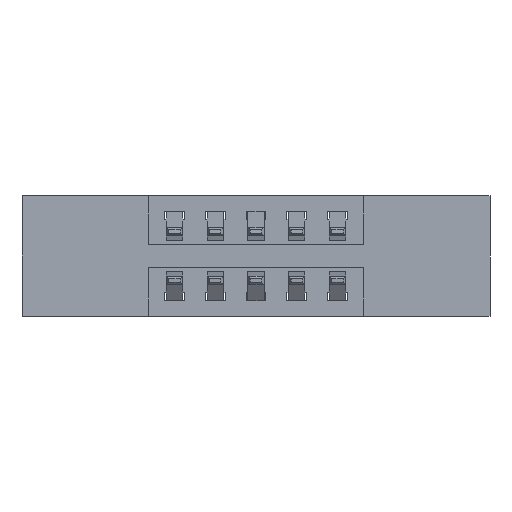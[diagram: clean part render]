
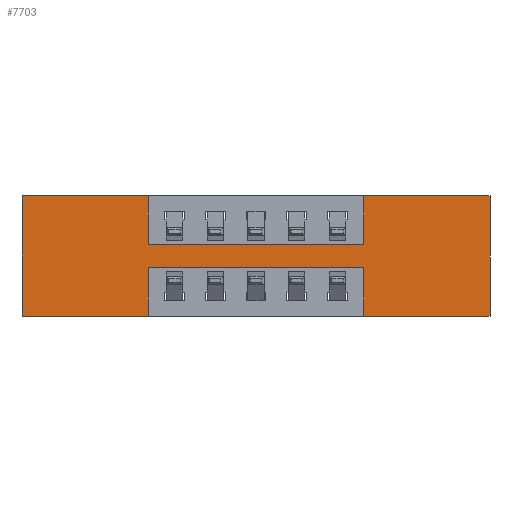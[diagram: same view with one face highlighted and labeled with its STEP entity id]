
A CAD part, front view. The second image highlights one B-rep face of the part: STEP entity #7703.
In plain terms, the highlighted planar face has unit normal (0, -1, 0).
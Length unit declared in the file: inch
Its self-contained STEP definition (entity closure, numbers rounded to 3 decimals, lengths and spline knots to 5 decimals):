
#15 = LINE ( 'NONE', #3158, #5585 ) ;
#16 = LINE ( 'NONE', #4874, #6699 ) ;
#152 = DIRECTION ( 'NONE',  ( 0., 0., 1. ) ) ;
#256 = EDGE_CURVE ( 'NONE', #5467, #5244, #16, .T. ) ;
#348 = ORIENTED_EDGE ( 'NONE', *, *, #256, .F. ) ;
#552 = CARTESIAN_POINT ( 'NONE',  ( 0.3875, 0., -0.22 ) ) ;
#829 = CARTESIAN_POINT ( 'NONE',  ( 0.3875, 0., 0. ) ) ;
#909 = LINE ( 'NONE', #829, #4134 ) ;
#952 = VERTEX_POINT ( 'NONE', #2493 ) ;
#1037 = DIRECTION ( 'NONE',  ( 1., 0., 0. ) ) ;
#1097 = ORIENTED_EDGE ( 'NONE', *, *, #2027, .F. ) ;
#1141 = CARTESIAN_POINT ( 'NONE',  ( 0., 0., 0. ) ) ;
#1165 = DIRECTION ( 'NONE',  ( -1., 0., 0. ) ) ;
#1270 = DIRECTION ( 'NONE',  ( 0., 0., -1. ) ) ;
#1451 = EDGE_CURVE ( 'NONE', #5244, #6331, #2304, .T. ) ;
#1646 = CARTESIAN_POINT ( 'NONE',  ( 0.3875, 0., -0.15 ) ) ;
#1742 = CARTESIAN_POINT ( 'NONE',  ( 0.3875, 0., -0.15 ) ) ;
#1752 = ORIENTED_EDGE ( 'NONE', *, *, #5271, .F. ) ;
#1842 = CARTESIAN_POINT ( 'NONE',  ( 1.435, 0., 0. ) ) ;
#1938 = CARTESIAN_POINT ( 'NONE',  ( 0., 0., -0.37 ) ) ;
#1953 = ORIENTED_EDGE ( 'NONE', *, *, #7779, .F. ) ;
#1957 = EDGE_LOOP ( 'NONE', ( #1752, #4332, #4628, #5695, #2259, #348, #4533, #7450, #1097, #2049, #7963, #1953 ) ) ;
#2027 = EDGE_CURVE ( 'NONE', #952, #4006, #909, .T. ) ;
#2049 = ORIENTED_EDGE ( 'NONE', *, *, #7031, .F. ) ;
#2076 = EDGE_CURVE ( 'NONE', #6331, #2893, #7748, .T. ) ;
#2101 = LINE ( 'NONE', #552, #5408 ) ;
#2259 = ORIENTED_EDGE ( 'NONE', *, *, #1451, .F. ) ;
#2304 = LINE ( 'NONE', #5465, #8083 ) ;
#2493 = CARTESIAN_POINT ( 'NONE',  ( 0.3875, 0., 0. ) ) ;
#2503 = DIRECTION ( 'NONE',  ( 0., -1., 0. ) ) ;
#2518 = LINE ( 'NONE', #1646, #4166 ) ;
#2599 = CARTESIAN_POINT ( 'NONE',  ( 0., 0., 0. ) ) ;
#2680 = CARTESIAN_POINT ( 'NONE',  ( 0., 0., -0.37 ) ) ;
#2754 = EDGE_CURVE ( 'NONE', #7626, #5467, #3765, .T. ) ;
#2893 = VERTEX_POINT ( 'NONE', #3043 ) ;
#2971 = VECTOR ( 'NONE', #152, 39.37008 ) ;
#3023 = CARTESIAN_POINT ( 'NONE',  ( 0.3875, 0., -0.22 ) ) ;
#3043 = CARTESIAN_POINT ( 'NONE',  ( 1.0475, 0., -0.37 ) ) ;
#3052 = DIRECTION ( 'NONE',  ( 0., 0., -1. ) ) ;
#3154 = CARTESIAN_POINT ( 'NONE',  ( 1.0475, 0., 0. ) ) ;
#3158 = CARTESIAN_POINT ( 'NONE',  ( 0., 0., -0.37 ) ) ;
#3169 = DIRECTION ( 'NONE',  ( 1., 0., 0. ) ) ;
#3387 = EDGE_CURVE ( 'NONE', #4006, #7626, #2518, .T. ) ;
#3481 = DIRECTION ( 'NONE',  ( 0., 0., -1. ) ) ;
#3765 = LINE ( 'NONE', #3154, #2971 ) ;
#3813 = EDGE_CURVE ( 'NONE', #2893, #7390, #5056, .T. ) ;
#3901 = VERTEX_POINT ( 'NONE', #6393 ) ;
#4006 = VERTEX_POINT ( 'NONE', #1742 ) ;
#4080 = DIRECTION ( 'NONE',  ( 0., 0., 1. ) ) ;
#4114 = VECTOR ( 'NONE', #7170, 39.37008 ) ;
#4128 = VECTOR ( 'NONE', #3481, 39.37008 ) ;
#4134 = VECTOR ( 'NONE', #3052, 39.37008 ) ;
#4166 = VECTOR ( 'NONE', #6750, 39.37008 ) ;
#4255 = VECTOR ( 'NONE', #4080, 39.37008 ) ;
#4318 = VECTOR ( 'NONE', #3169, 39.37008 ) ;
#4332 = ORIENTED_EDGE ( 'NONE', *, *, #5857, .F. ) ;
#4336 = LINE ( 'NONE', #8113, #4128 ) ;
#4382 = FACE_OUTER_BOUND ( 'NONE', #1957, .T. ) ;
#4533 = ORIENTED_EDGE ( 'NONE', *, *, #2754, .F. ) ;
#4628 = ORIENTED_EDGE ( 'NONE', *, *, #3813, .F. ) ;
#4759 = CARTESIAN_POINT ( 'NONE',  ( 1.435, 0., -0.37 ) ) ;
#4863 = CARTESIAN_POINT ( 'NONE',  ( 0., 0., 0. ) ) ;
#4874 = CARTESIAN_POINT ( 'NONE',  ( 0., 0., 0. ) ) ;
#4941 = VERTEX_POINT ( 'NONE', #3023 ) ;
#5006 = VERTEX_POINT ( 'NONE', #1141 ) ;
#5056 = LINE ( 'NONE', #6075, #4255 ) ;
#5075 = CARTESIAN_POINT ( 'NONE',  ( 0., 0., -0.37 ) ) ;
#5244 = VERTEX_POINT ( 'NONE', #1842 ) ;
#5271 = EDGE_CURVE ( 'NONE', #4941, #3901, #4336, .T. ) ;
#5408 = VECTOR ( 'NONE', #5653, 39.37008 ) ;
#5436 = DIRECTION ( 'NONE',  ( 0., 0., 1. ) ) ;
#5465 = CARTESIAN_POINT ( 'NONE',  ( 1.435, 0., 0. ) ) ;
#5467 = VERTEX_POINT ( 'NONE', #6349 ) ;
#5585 = VECTOR ( 'NONE', #1165, 39.37008 ) ;
#5653 = DIRECTION ( 'NONE',  ( -1., 0., 0. ) ) ;
#5667 = PLANE ( 'NONE',  #7977 ) ;
#5695 = ORIENTED_EDGE ( 'NONE', *, *, #2076, .F. ) ;
#5857 = EDGE_CURVE ( 'NONE', #7390, #4941, #2101, .T. ) ;
#5869 = VERTEX_POINT ( 'NONE', #5075 ) ;
#6075 = CARTESIAN_POINT ( 'NONE',  ( 1.0475, 0., -0.37 ) ) ;
#6229 = LINE ( 'NONE', #2599, #4318 ) ;
#6331 = VERTEX_POINT ( 'NONE', #4759 ) ;
#6349 = CARTESIAN_POINT ( 'NONE',  ( 1.0475, 0., 0. ) ) ;
#6393 = CARTESIAN_POINT ( 'NONE',  ( 0.3875, 0., -0.37 ) ) ;
#6445 = EDGE_CURVE ( 'NONE', #5869, #5006, #7246, .T. ) ;
#6699 = VECTOR ( 'NONE', #1037, 39.37008 ) ;
#6750 = DIRECTION ( 'NONE',  ( 1., 0., 0. ) ) ;
#6784 = CARTESIAN_POINT ( 'NONE',  ( 1.0475, 0., -0.22 ) ) ;
#7031 = EDGE_CURVE ( 'NONE', #5006, #952, #6229, .T. ) ;
#7170 = DIRECTION ( 'NONE',  ( -1., 0., 0. ) ) ;
#7246 = LINE ( 'NONE', #4863, #7776 ) ;
#7390 = VERTEX_POINT ( 'NONE', #6784 ) ;
#7450 = ORIENTED_EDGE ( 'NONE', *, *, #3387, .F. ) ;
#7626 = VERTEX_POINT ( 'NONE', #8034 ) ;
#7703 = ADVANCED_FACE ( 'NONE', ( #4382 ), #5667, .T. ) ;
#7748 = LINE ( 'NONE', #2680, #4114 ) ;
#7776 = VECTOR ( 'NONE', #5436, 39.37008 ) ;
#7779 = EDGE_CURVE ( 'NONE', #3901, #5869, #15, .T. ) ;
#7963 = ORIENTED_EDGE ( 'NONE', *, *, #6445, .F. ) ;
#7964 = DIRECTION ( 'NONE',  ( 0., 0., -1. ) ) ;
#7977 = AXIS2_PLACEMENT_3D ( 'NONE', #1938, #2503, #1270 ) ;
#8034 = CARTESIAN_POINT ( 'NONE',  ( 1.0475, 0., -0.15 ) ) ;
#8083 = VECTOR ( 'NONE', #7964, 39.37008 ) ;
#8113 = CARTESIAN_POINT ( 'NONE',  ( 0.3875, 0., -0.37 ) ) ;
